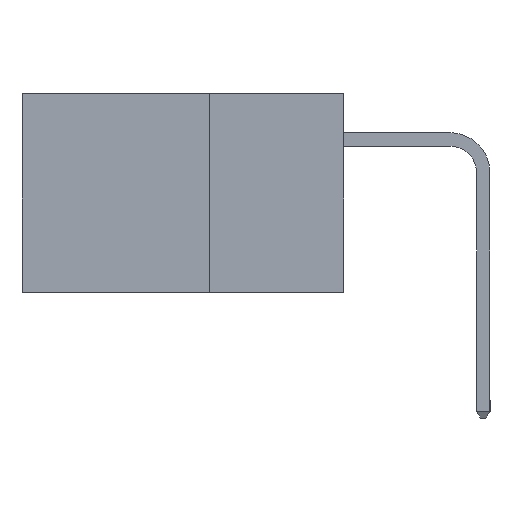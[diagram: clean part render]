
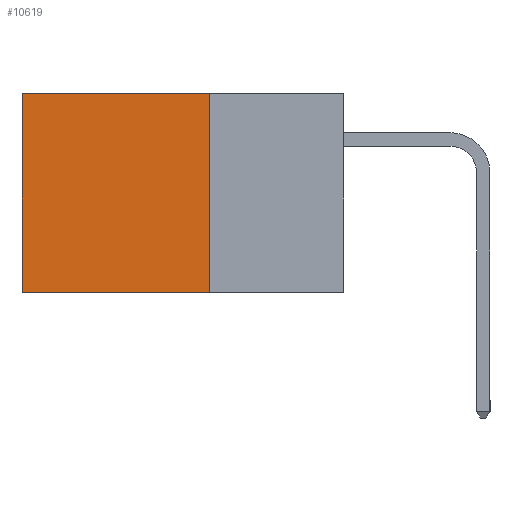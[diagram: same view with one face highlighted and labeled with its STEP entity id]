
A CAD part, left-side view. The second image highlights one B-rep face of the part: STEP entity #10619.
In plain terms, the highlighted planar face has unit normal (-1, 0, 0).
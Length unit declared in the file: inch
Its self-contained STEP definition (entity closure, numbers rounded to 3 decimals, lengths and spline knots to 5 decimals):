
#258 = CARTESIAN_POINT ( 'NONE',  ( 0.2615, 0.6, -0.37 ) ) ;
#1081 = CARTESIAN_POINT ( 'NONE',  ( 0.2615, 0.25, -0.37 ) ) ;
#2269 = DIRECTION ( 'NONE',  ( 0., 0., -1. ) ) ;
#2321 = CARTESIAN_POINT ( 'NONE',  ( 0.2615, 0.25, -0.37 ) ) ;
#2813 = VERTEX_POINT ( 'NONE', #13339 ) ;
#3876 = VERTEX_POINT ( 'NONE', #7840 ) ;
#3919 = EDGE_CURVE ( 'NONE', #9279, #2813, #7164, .T. ) ;
#4105 = EDGE_CURVE ( 'NONE', #3876, #7345, #4207, .T. ) ;
#4207 = LINE ( 'NONE', #16183, #14418 ) ;
#4450 = LINE ( 'NONE', #2321, #7602 ) ;
#5546 = DIRECTION ( 'NONE',  ( 0., 1., 0. ) ) ;
#5997 = ORIENTED_EDGE ( 'NONE', *, *, #11094, .T. ) ;
#6150 = CARTESIAN_POINT ( 'NONE',  ( 0.2615, 0.25, -0.37 ) ) ;
#6548 = CARTESIAN_POINT ( 'NONE',  ( 0.2615, 0.6, 0. ) ) ;
#6741 = VECTOR ( 'NONE', #9220, 39.37008 ) ;
#6742 = AXIS2_PLACEMENT_3D ( 'NONE', #6150, #15417, #7497 ) ;
#7164 = LINE ( 'NONE', #1081, #6741 ) ;
#7345 = VERTEX_POINT ( 'NONE', #6548 ) ;
#7497 = DIRECTION ( 'NONE',  ( 0., 0., -1. ) ) ;
#7602 = VECTOR ( 'NONE', #13084, 39.37008 ) ;
#7840 = CARTESIAN_POINT ( 'NONE',  ( 0.2615, 0.25, 0. ) ) ;
#9220 = DIRECTION ( 'NONE',  ( 0., 1., 0. ) ) ;
#9279 = VERTEX_POINT ( 'NONE', #14613 ) ;
#9325 = ORIENTED_EDGE ( 'NONE', *, *, #15006, .F. ) ;
#10019 = VECTOR ( 'NONE', #2269, 39.37008 ) ;
#10619 = ADVANCED_FACE ( 'NONE', ( #12894 ), #14111, .F. ) ;
#11094 = EDGE_CURVE ( 'NONE', #7345, #2813, #13512, .T. ) ;
#11285 = EDGE_LOOP ( 'NONE', ( #5997, #12160, #9325, #11311 ) ) ;
#11311 = ORIENTED_EDGE ( 'NONE', *, *, #4105, .T. ) ;
#12160 = ORIENTED_EDGE ( 'NONE', *, *, #3919, .F. ) ;
#12894 = FACE_OUTER_BOUND ( 'NONE', #11285, .T. ) ;
#13084 = DIRECTION ( 'NONE',  ( 0., 0., -1. ) ) ;
#13339 = CARTESIAN_POINT ( 'NONE',  ( 0.2615, 0.6, -0.37 ) ) ;
#13512 = LINE ( 'NONE', #258, #10019 ) ;
#14111 = PLANE ( 'NONE',  #6742 ) ;
#14418 = VECTOR ( 'NONE', #5546, 39.37008 ) ;
#14613 = CARTESIAN_POINT ( 'NONE',  ( 0.2615, 0.25, -0.37 ) ) ;
#15006 = EDGE_CURVE ( 'NONE', #3876, #9279, #4450, .T. ) ;
#15417 = DIRECTION ( 'NONE',  ( 1., 0., 0. ) ) ;
#16183 = CARTESIAN_POINT ( 'NONE',  ( 0.2615, 0.25, 0. ) ) ;
